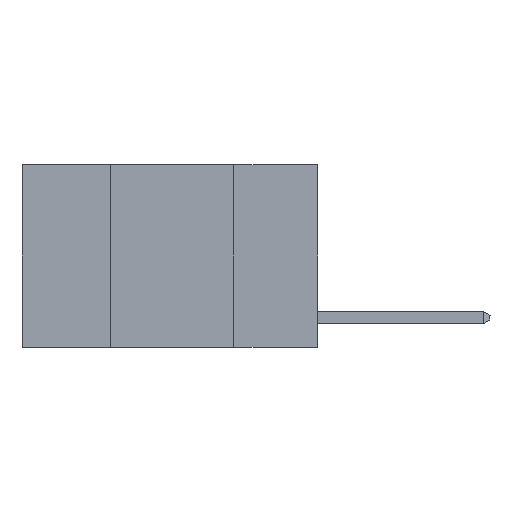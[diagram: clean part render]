
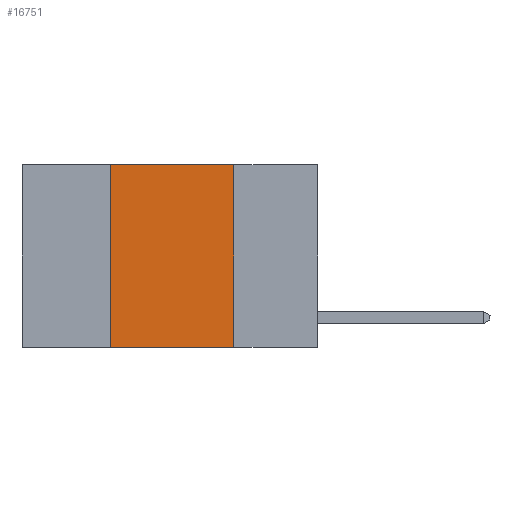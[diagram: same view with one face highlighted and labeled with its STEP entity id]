
A CAD part, left-side view. The second image highlights one B-rep face of the part: STEP entity #16751.
In plain terms, the highlighted planar face has unit normal (-1, 0, 0).
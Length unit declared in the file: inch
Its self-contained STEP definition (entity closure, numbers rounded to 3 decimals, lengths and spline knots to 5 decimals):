
#1283 = CARTESIAN_POINT ( 'NONE',  ( 0., 0.6, -0.37 ) ) ;
#1753 = VERTEX_POINT ( 'NONE', #20289 ) ;
#1759 = VECTOR ( 'NONE', #14834, 39.37008 ) ;
#1764 = DIRECTION ( 'NONE',  ( 1., 0., 0. ) ) ;
#1974 = ORIENTED_EDGE ( 'NONE', *, *, #4272, .T. ) ;
#3212 = AXIS2_PLACEMENT_3D ( 'NONE', #27346, #1764, #16719 ) ;
#3785 = CARTESIAN_POINT ( 'NONE',  ( 0., 0.42, -0.37 ) ) ;
#4272 = EDGE_CURVE ( 'NONE', #22964, #10195, #27642, .T. ) ;
#5613 = DIRECTION ( 'NONE',  ( 0., -1., 0. ) ) ;
#7272 = ORIENTED_EDGE ( 'NONE', *, *, #10613, .F. ) ;
#8188 = ORIENTED_EDGE ( 'NONE', *, *, #12751, .F. ) ;
#8554 = EDGE_CURVE ( 'NONE', #1753, #10195, #16937, .T. ) ;
#8927 = VERTEX_POINT ( 'NONE', #17473 ) ;
#9739 = LINE ( 'NONE', #22423, #14031 ) ;
#10195 = VERTEX_POINT ( 'NONE', #26179 ) ;
#10613 = EDGE_CURVE ( 'NONE', #22964, #8927, #23837, .T. ) ;
#10643 = VECTOR ( 'NONE', #5613, 39.37008 ) ;
#12422 = PLANE ( 'NONE',  #3212 ) ;
#12751 = EDGE_CURVE ( 'NONE', #8927, #1753, #9739, .T. ) ;
#13803 = DIRECTION ( 'NONE',  ( 0., -1., 0. ) ) ;
#14031 = VECTOR ( 'NONE', #13803, 39.37008 ) ;
#14669 = CARTESIAN_POINT ( 'NONE',  ( 0., 0.17, 0. ) ) ;
#14834 = DIRECTION ( 'NONE',  ( 0., 0., 1. ) ) ;
#16719 = DIRECTION ( 'NONE',  ( 0., 0., -1. ) ) ;
#16751 = ADVANCED_FACE ( 'NONE', ( #19389 ), #12422, .F. ) ;
#16937 = LINE ( 'NONE', #14669, #21265 ) ;
#17473 = CARTESIAN_POINT ( 'NONE',  ( 0., 0.42, 0. ) ) ;
#19389 = FACE_OUTER_BOUND ( 'NONE', #23776, .T. ) ;
#20289 = CARTESIAN_POINT ( 'NONE',  ( 0., 0.17, 0. ) ) ;
#21265 = VECTOR ( 'NONE', #27484, 39.37008 ) ;
#21598 = ORIENTED_EDGE ( 'NONE', *, *, #8554, .F. ) ;
#22423 = CARTESIAN_POINT ( 'NONE',  ( 0., 0.6, 0. ) ) ;
#22964 = VERTEX_POINT ( 'NONE', #3785 ) ;
#23776 = EDGE_LOOP ( 'NONE', ( #21598, #8188, #7272, #1974 ) ) ;
#23837 = LINE ( 'NONE', #27641, #1759 ) ;
#26179 = CARTESIAN_POINT ( 'NONE',  ( 0., 0.17, -0.37 ) ) ;
#27346 = CARTESIAN_POINT ( 'NONE',  ( 0., 0.6, 0. ) ) ;
#27484 = DIRECTION ( 'NONE',  ( 0., 0., -1. ) ) ;
#27641 = CARTESIAN_POINT ( 'NONE',  ( 0., 0.42, 0. ) ) ;
#27642 = LINE ( 'NONE', #1283, #10643 ) ;
